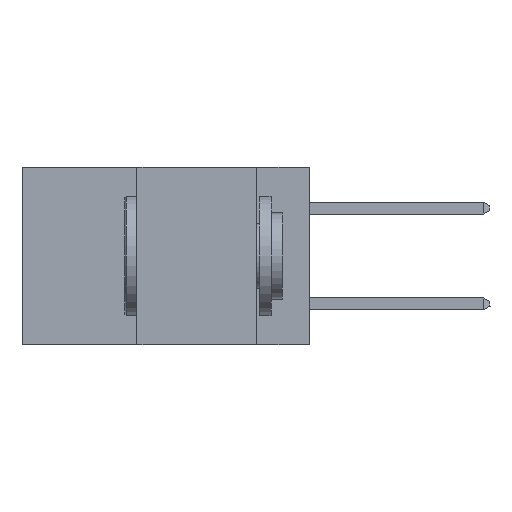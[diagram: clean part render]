
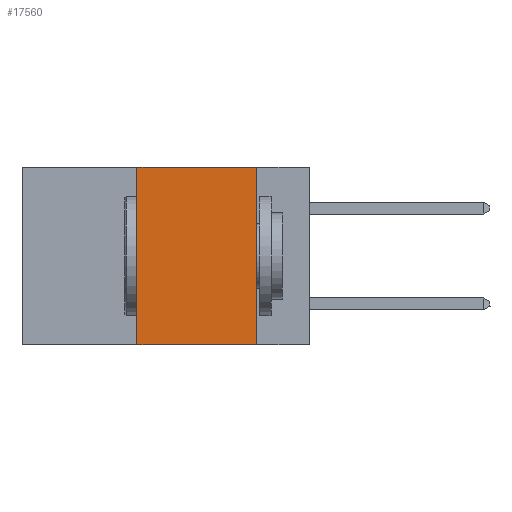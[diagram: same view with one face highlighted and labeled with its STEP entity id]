
A CAD part, left-side view. The second image highlights one B-rep face of the part: STEP entity #17560.
In plain terms, the highlighted planar face has unit normal (-1, 0, 0).
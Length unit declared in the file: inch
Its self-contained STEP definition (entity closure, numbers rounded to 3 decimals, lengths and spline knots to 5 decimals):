
#582 = DIRECTION ( 'NONE',  ( 0., 0., 1. ) ) ;
#2306 = DIRECTION ( 'NONE',  ( 0., 0., -1. ) ) ;
#2919 = CARTESIAN_POINT ( 'NONE',  ( 0., 0.6, 0. ) ) ;
#3047 = CARTESIAN_POINT ( 'NONE',  ( 0., 0.11, -0.37 ) ) ;
#3295 = LINE ( 'NONE', #7079, #4586 ) ;
#4586 = VECTOR ( 'NONE', #9507, 39.37008 ) ;
#4605 = AXIS2_PLACEMENT_3D ( 'NONE', #2919, #30443, #9457 ) ;
#5562 = VECTOR ( 'NONE', #11663, 39.37008 ) ;
#5659 = EDGE_CURVE ( 'NONE', #35992, #23709, #16570, .T. ) ;
#5830 = CARTESIAN_POINT ( 'NONE',  ( 0., 0.36, 0. ) ) ;
#7079 = CARTESIAN_POINT ( 'NONE',  ( 0., 0.6, -0.37 ) ) ;
#8875 = CARTESIAN_POINT ( 'NONE',  ( 0., 0.6, 0. ) ) ;
#9457 = DIRECTION ( 'NONE',  ( 0., 0., -1. ) ) ;
#9507 = DIRECTION ( 'NONE',  ( 0., -1., 0. ) ) ;
#10076 = ORIENTED_EDGE ( 'NONE', *, *, #5659, .F. ) ;
#11663 = DIRECTION ( 'NONE',  ( 0., -1., 0. ) ) ;
#11723 = EDGE_LOOP ( 'NONE', ( #10076, #20265, #14826, #24516 ) ) ;
#13710 = CARTESIAN_POINT ( 'NONE',  ( 0., 0.36, 0. ) ) ;
#14826 = ORIENTED_EDGE ( 'NONE', *, *, #28135, .F. ) ;
#15278 = FACE_OUTER_BOUND ( 'NONE', #11723, .T. ) ;
#16570 = LINE ( 'NONE', #19204, #23177 ) ;
#17560 = ADVANCED_FACE ( 'NONE', ( #15278 ), #30152, .F. ) ;
#18984 = EDGE_CURVE ( 'NONE', #22319, #35992, #33736, .T. ) ;
#19204 = CARTESIAN_POINT ( 'NONE',  ( 0., 0.11, 0. ) ) ;
#19604 = LINE ( 'NONE', #5830, #31087 ) ;
#20265 = ORIENTED_EDGE ( 'NONE', *, *, #18984, .F. ) ;
#22319 = VERTEX_POINT ( 'NONE', #13710 ) ;
#23049 = EDGE_CURVE ( 'NONE', #32262, #23709, #3295, .T. ) ;
#23177 = VECTOR ( 'NONE', #2306, 39.37008 ) ;
#23709 = VERTEX_POINT ( 'NONE', #3047 ) ;
#24516 = ORIENTED_EDGE ( 'NONE', *, *, #23049, .T. ) ;
#24969 = CARTESIAN_POINT ( 'NONE',  ( 0., 0.36, -0.37 ) ) ;
#28135 = EDGE_CURVE ( 'NONE', #32262, #22319, #19604, .T. ) ;
#28854 = CARTESIAN_POINT ( 'NONE',  ( 0., 0.11, 0. ) ) ;
#30152 = PLANE ( 'NONE',  #4605 ) ;
#30443 = DIRECTION ( 'NONE',  ( 1., 0., 0. ) ) ;
#31087 = VECTOR ( 'NONE', #582, 39.37008 ) ;
#32262 = VERTEX_POINT ( 'NONE', #24969 ) ;
#33736 = LINE ( 'NONE', #8875, #5562 ) ;
#35992 = VERTEX_POINT ( 'NONE', #28854 ) ;
